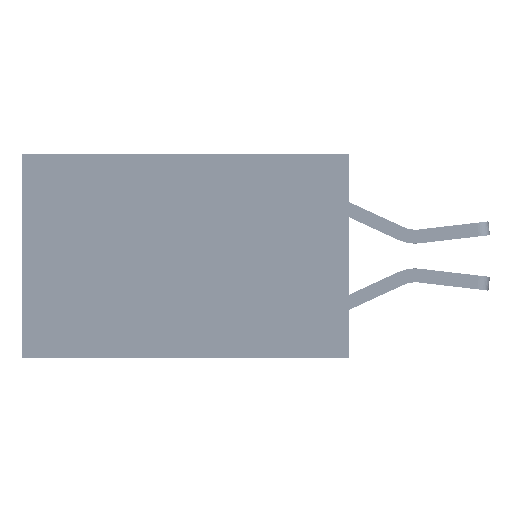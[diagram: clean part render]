
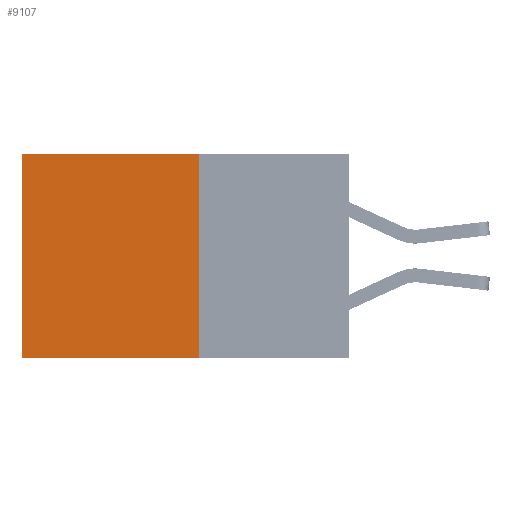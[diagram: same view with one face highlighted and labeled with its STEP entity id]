
A CAD part, left-side view. The second image highlights one B-rep face of the part: STEP entity #9107.
In plain terms, the highlighted planar face has unit normal (-1, 0, 0).
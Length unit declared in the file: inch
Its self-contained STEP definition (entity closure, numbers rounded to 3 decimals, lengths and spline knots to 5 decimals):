
#1628 = PLANE ( 'NONE',  #35816 ) ;
#2691 = VECTOR ( 'NONE', #33473, 39.37008 ) ;
#3574 = LINE ( 'NONE', #16868, #2691 ) ;
#4449 = DIRECTION ( 'NONE',  ( 0., 0., -1. ) ) ;
#5183 = CARTESIAN_POINT ( 'NONE',  ( 0.277, 0.27, 0. ) ) ;
#5583 = DIRECTION ( 'NONE',  ( 0., 1., 0. ) ) ;
#6723 = VERTEX_POINT ( 'NONE', #7916 ) ;
#7216 = ORIENTED_EDGE ( 'NONE', *, *, #16049, .F. ) ;
#7916 = CARTESIAN_POINT ( 'NONE',  ( 0.277, 0.27, 0. ) ) ;
#8539 = DIRECTION ( 'NONE',  ( 0., 0., -1. ) ) ;
#9025 = CARTESIAN_POINT ( 'NONE',  ( 0.277, 0.59, 0. ) ) ;
#9107 = ADVANCED_FACE ( 'NONE', ( #17701 ), #1628, .F. ) ;
#9550 = VERTEX_POINT ( 'NONE', #9025 ) ;
#11259 = CARTESIAN_POINT ( 'NONE',  ( 0.277, 0.59, -0.37 ) ) ;
#13050 = CARTESIAN_POINT ( 'NONE',  ( 0.277, 0.27, -0.37 ) ) ;
#13689 = VECTOR ( 'NONE', #8539, 39.37008 ) ;
#13741 = EDGE_CURVE ( 'NONE', #6723, #9550, #33494, .T. ) ;
#13781 = VERTEX_POINT ( 'NONE', #22555 ) ;
#13893 = ORIENTED_EDGE ( 'NONE', *, *, #30725, .T. ) ;
#15430 = LINE ( 'NONE', #11259, #13689 ) ;
#16049 = EDGE_CURVE ( 'NONE', #6723, #32949, #32481, .T. ) ;
#16868 = CARTESIAN_POINT ( 'NONE',  ( 0.277, 0.27, -0.37 ) ) ;
#17701 = FACE_OUTER_BOUND ( 'NONE', #21089, .T. ) ;
#18425 = CARTESIAN_POINT ( 'NONE',  ( 0.277, 0.27, -0.37 ) ) ;
#18735 = VECTOR ( 'NONE', #5583, 39.37008 ) ;
#21089 = EDGE_LOOP ( 'NONE', ( #13893, #25672, #7216, #25153 ) ) ;
#21223 = DIRECTION ( 'NONE',  ( 1., 0., 0. ) ) ;
#22555 = CARTESIAN_POINT ( 'NONE',  ( 0.277, 0.59, -0.37 ) ) ;
#25153 = ORIENTED_EDGE ( 'NONE', *, *, #13741, .T. ) ;
#25672 = ORIENTED_EDGE ( 'NONE', *, *, #27989, .F. ) ;
#27989 = EDGE_CURVE ( 'NONE', #32949, #13781, #3574, .T. ) ;
#30725 = EDGE_CURVE ( 'NONE', #9550, #13781, #15430, .T. ) ;
#32472 = DIRECTION ( 'NONE',  ( 0., 0., -1. ) ) ;
#32478 = CARTESIAN_POINT ( 'NONE',  ( 0.277, 0.27, -0.37 ) ) ;
#32481 = LINE ( 'NONE', #13050, #34176 ) ;
#32949 = VERTEX_POINT ( 'NONE', #32478 ) ;
#33473 = DIRECTION ( 'NONE',  ( 0., 1., 0. ) ) ;
#33494 = LINE ( 'NONE', #5183, #18735 ) ;
#34176 = VECTOR ( 'NONE', #32472, 39.37008 ) ;
#35816 = AXIS2_PLACEMENT_3D ( 'NONE', #18425, #21223, #4449 ) ;
